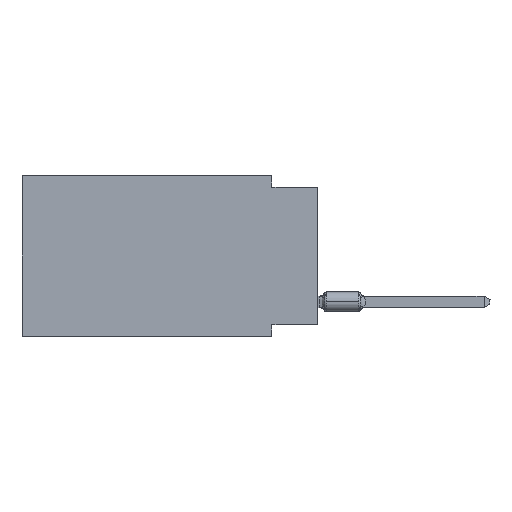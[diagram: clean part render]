
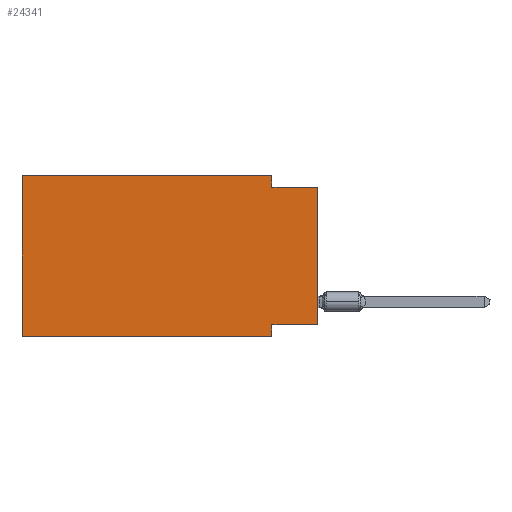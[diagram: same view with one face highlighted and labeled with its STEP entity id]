
A CAD part, left-side view. The second image highlights one B-rep face of the part: STEP entity #24341.
In plain terms, the highlighted planar face has unit normal (-1, 0, 0).
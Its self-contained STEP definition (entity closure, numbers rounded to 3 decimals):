
#1604 = VERTEX_POINT ( 'NONE', #4207 ) ;
#2082 = CARTESIAN_POINT ( 'NONE',  ( 0., 2.54, -8.255 ) ) ;
#2574 = DIRECTION ( 'NONE',  ( 0., -1., 0. ) ) ;
#3206 = VECTOR ( 'NONE', #47337, 1000. ) ;
#3235 = CARTESIAN_POINT ( 'NONE',  ( 0., 0., -0.635 ) ) ;
#4207 = CARTESIAN_POINT ( 'NONE',  ( 0., 2.54, 0. ) ) ;
#4629 = CARTESIAN_POINT ( 'NONE',  ( 0., 0., -0.635 ) ) ;
#5095 = ORIENTED_EDGE ( 'NONE', *, *, #40584, .T. ) ;
#5915 = EDGE_CURVE ( 'NONE', #14553, #39739, #13121, .T. ) ;
#6072 = VECTOR ( 'NONE', #9344, 1000. ) ;
#7354 = VECTOR ( 'NONE', #2574, 1000. ) ;
#7771 = ORIENTED_EDGE ( 'NONE', *, *, #42846, .F. ) ;
#9177 = CARTESIAN_POINT ( 'NONE',  ( 0., 16.383, -8.89 ) ) ;
#9344 = DIRECTION ( 'NONE',  ( 0., 0., -1. ) ) ;
#9624 = LINE ( 'NONE', #17640, #7354 ) ;
#9966 = CARTESIAN_POINT ( 'NONE',  ( 0., 16.383, 0. ) ) ;
#10287 = DIRECTION ( 'NONE',  ( 0., -1., 0. ) ) ;
#11164 = EDGE_CURVE ( 'NONE', #25021, #26294, #39106, .T. ) ;
#11904 = EDGE_CURVE ( 'NONE', #37533, #31509, #23077, .T. ) ;
#12202 = LINE ( 'NONE', #9177, #3206 ) ;
#13121 = LINE ( 'NONE', #28429, #6072 ) ;
#14553 = VERTEX_POINT ( 'NONE', #2082 ) ;
#14556 = VECTOR ( 'NONE', #42947, 1000. ) ;
#16130 = VECTOR ( 'NONE', #24566, 1000. ) ;
#16942 = ORIENTED_EDGE ( 'NONE', *, *, #33600, .F. ) ;
#17640 = CARTESIAN_POINT ( 'NONE',  ( 0., 16.383, 0. ) ) ;
#19633 = AXIS2_PLACEMENT_3D ( 'NONE', #46040, #37521, #25962 ) ;
#20445 = ORIENTED_EDGE ( 'NONE', *, *, #32782, .F. ) ;
#22182 = PLANE ( 'NONE',  #19633 ) ;
#23077 = LINE ( 'NONE', #27621, #14556 ) ;
#24341 = ADVANCED_FACE ( 'NONE', ( #30734 ), #22182, .F. ) ;
#24566 = DIRECTION ( 'NONE',  ( 0., 1., 0. ) ) ;
#25021 = VERTEX_POINT ( 'NONE', #39687 ) ;
#25314 = LINE ( 'NONE', #39901, #16130 ) ;
#25837 = VERTEX_POINT ( 'NONE', #39363 ) ;
#25962 = DIRECTION ( 'NONE',  ( 0., 0., -1. ) ) ;
#26294 = VERTEX_POINT ( 'NONE', #4629 ) ;
#26984 = DIRECTION ( 'NONE',  ( 0., 0., -1. ) ) ;
#27416 = VECTOR ( 'NONE', #10287, 1000. ) ;
#27597 = ORIENTED_EDGE ( 'NONE', *, *, #11904, .F. ) ;
#27621 = CARTESIAN_POINT ( 'NONE',  ( 0., 16.383, 0. ) ) ;
#28429 = CARTESIAN_POINT ( 'NONE',  ( 0., 2.54, -8.89 ) ) ;
#28548 = CARTESIAN_POINT ( 'NONE',  ( 0., 0., 0. ) ) ;
#30370 = LINE ( 'NONE', #3235, #27416 ) ;
#30734 = FACE_OUTER_BOUND ( 'NONE', #43860, .T. ) ;
#31509 = VERTEX_POINT ( 'NONE', #9966 ) ;
#32540 = ORIENTED_EDGE ( 'NONE', *, *, #11164, .T. ) ;
#32782 = EDGE_CURVE ( 'NONE', #31509, #1604, #9624, .T. ) ;
#33600 = EDGE_CURVE ( 'NONE', #25021, #14553, #25314, .T. ) ;
#34043 = LINE ( 'NONE', #49344, #38561 ) ;
#37326 = VECTOR ( 'NONE', #39852, 1000. ) ;
#37521 = DIRECTION ( 'NONE',  ( 1., 0., 0. ) ) ;
#37533 = VERTEX_POINT ( 'NONE', #45322 ) ;
#37562 = EDGE_CURVE ( 'NONE', #1604, #25837, #34043, .T. ) ;
#38561 = VECTOR ( 'NONE', #26984, 1000. ) ;
#39106 = LINE ( 'NONE', #28548, #37326 ) ;
#39363 = CARTESIAN_POINT ( 'NONE',  ( 0., 2.54, -0.635 ) ) ;
#39687 = CARTESIAN_POINT ( 'NONE',  ( 0., 0., -8.255 ) ) ;
#39739 = VERTEX_POINT ( 'NONE', #42511 ) ;
#39852 = DIRECTION ( 'NONE',  ( 0., 0., 1. ) ) ;
#39901 = CARTESIAN_POINT ( 'NONE',  ( 0., 0., -8.255 ) ) ;
#40584 = EDGE_CURVE ( 'NONE', #37533, #39739, #12202, .T. ) ;
#42511 = CARTESIAN_POINT ( 'NONE',  ( 0., 2.54, -8.89 ) ) ;
#42846 = EDGE_CURVE ( 'NONE', #25837, #26294, #30370, .T. ) ;
#42947 = DIRECTION ( 'NONE',  ( 0., 0., 1. ) ) ;
#43528 = ORIENTED_EDGE ( 'NONE', *, *, #37562, .F. ) ;
#43860 = EDGE_LOOP ( 'NONE', ( #32540, #7771, #43528, #20445, #27597, #5095, #45667, #16942 ) ) ;
#45322 = CARTESIAN_POINT ( 'NONE',  ( 0., 16.383, -8.89 ) ) ;
#45667 = ORIENTED_EDGE ( 'NONE', *, *, #5915, .F. ) ;
#46040 = CARTESIAN_POINT ( 'NONE',  ( 0., 16.383, 0. ) ) ;
#47337 = DIRECTION ( 'NONE',  ( 0., -1., 0. ) ) ;
#49344 = CARTESIAN_POINT ( 'NONE',  ( 0., 2.54, 0. ) ) ;
